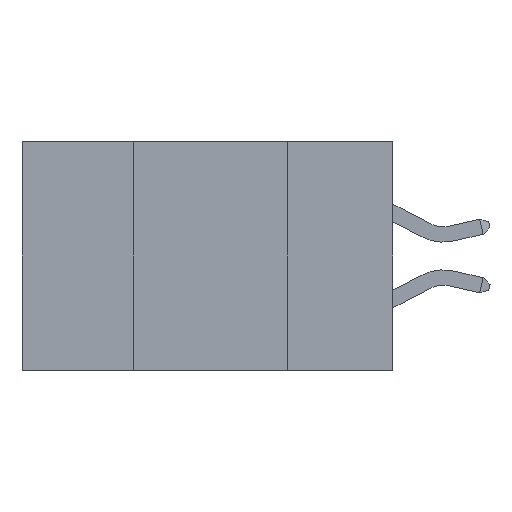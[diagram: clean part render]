
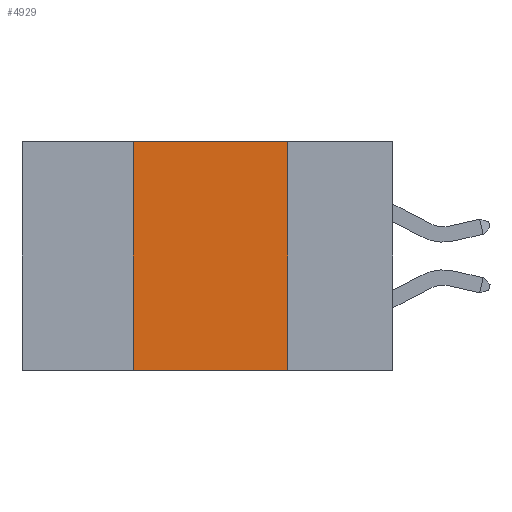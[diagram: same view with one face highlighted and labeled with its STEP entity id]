
A CAD part, left-side view. The second image highlights one B-rep face of the part: STEP entity #4929.
In plain terms, the highlighted planar face has unit normal (-1, 0, 0).
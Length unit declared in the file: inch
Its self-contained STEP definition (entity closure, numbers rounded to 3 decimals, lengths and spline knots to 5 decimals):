
#301 = CARTESIAN_POINT ( 'NONE',  ( 0., 0.6, 0. ) ) ;
#986 = VERTEX_POINT ( 'NONE', #27641 ) ;
#2094 = DIRECTION ( 'NONE',  ( 0., -1., 0. ) ) ;
#2939 = EDGE_CURVE ( 'NONE', #28994, #7996, #30718, .T. ) ;
#4485 = VERTEX_POINT ( 'NONE', #28148 ) ;
#4929 = ADVANCED_FACE ( 'NONE', ( #26129 ), #27853, .F. ) ;
#6925 = DIRECTION ( 'NONE',  ( 0., 0., -1. ) ) ;
#7113 = EDGE_CURVE ( 'NONE', #28994, #986, #30470, .T. ) ;
#7159 = CARTESIAN_POINT ( 'NONE',  ( 0., 0.17, 0. ) ) ;
#7173 = VECTOR ( 'NONE', #2094, 39.37008 ) ;
#7764 = ORIENTED_EDGE ( 'NONE', *, *, #2939, .F. ) ;
#7996 = VERTEX_POINT ( 'NONE', #29607 ) ;
#8125 = DIRECTION ( 'NONE',  ( 0., -1., 0. ) ) ;
#8271 = CARTESIAN_POINT ( 'NONE',  ( 0., 0.42, 0. ) ) ;
#9373 = DIRECTION ( 'NONE',  ( 0., 0., 1. ) ) ;
#9667 = ORIENTED_EDGE ( 'NONE', *, *, #16527, .F. ) ;
#9681 = ORIENTED_EDGE ( 'NONE', *, *, #7113, .T. ) ;
#9829 = ORIENTED_EDGE ( 'NONE', *, *, #12336, .F. ) ;
#12336 = EDGE_CURVE ( 'NONE', #4485, #986, #12697, .T. ) ;
#12697 = LINE ( 'NONE', #7159, #29883 ) ;
#14223 = AXIS2_PLACEMENT_3D ( 'NONE', #30228, #14588, #32836 ) ;
#14588 = DIRECTION ( 'NONE',  ( 1., 0., 0. ) ) ;
#16527 = EDGE_CURVE ( 'NONE', #7996, #4485, #23332, .T. ) ;
#17223 = VECTOR ( 'NONE', #8125, 39.37008 ) ;
#20266 = CARTESIAN_POINT ( 'NONE',  ( 0., 0.6, -0.37 ) ) ;
#20341 = CARTESIAN_POINT ( 'NONE',  ( 0., 0.42, -0.37 ) ) ;
#23332 = LINE ( 'NONE', #301, #17223 ) ;
#26129 = FACE_OUTER_BOUND ( 'NONE', #26466, .T. ) ;
#26466 = EDGE_LOOP ( 'NONE', ( #9829, #9667, #7764, #9681 ) ) ;
#27641 = CARTESIAN_POINT ( 'NONE',  ( 0., 0.17, -0.37 ) ) ;
#27853 = PLANE ( 'NONE',  #14223 ) ;
#28148 = CARTESIAN_POINT ( 'NONE',  ( 0., 0.17, 0. ) ) ;
#28994 = VERTEX_POINT ( 'NONE', #20341 ) ;
#29607 = CARTESIAN_POINT ( 'NONE',  ( 0., 0.42, 0. ) ) ;
#29883 = VECTOR ( 'NONE', #6925, 39.37008 ) ;
#30228 = CARTESIAN_POINT ( 'NONE',  ( 0., 0.6, 0. ) ) ;
#30470 = LINE ( 'NONE', #20266, #7173 ) ;
#30718 = LINE ( 'NONE', #8271, #31527 ) ;
#31527 = VECTOR ( 'NONE', #9373, 39.37008 ) ;
#32836 = DIRECTION ( 'NONE',  ( 0., 0., -1. ) ) ;
